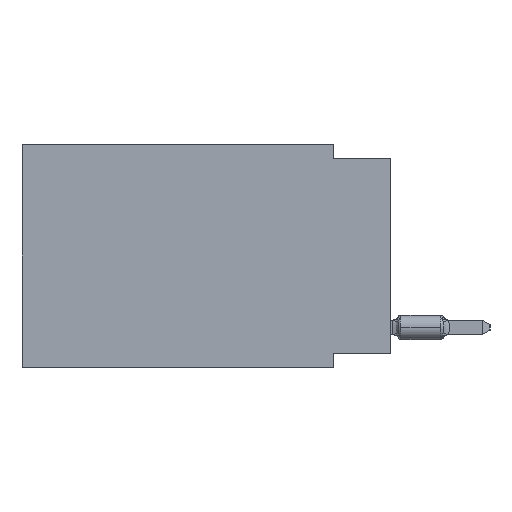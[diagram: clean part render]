
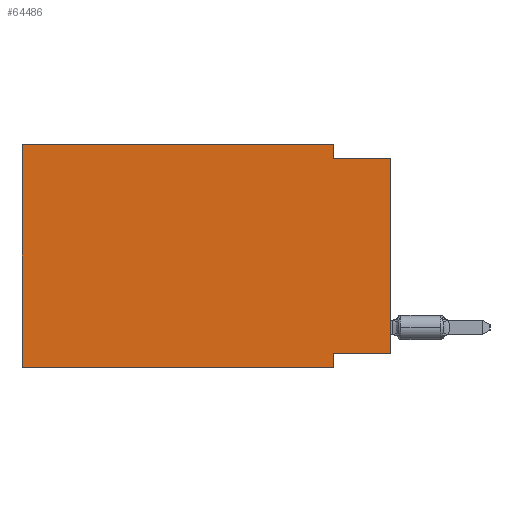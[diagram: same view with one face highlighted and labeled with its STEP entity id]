
A CAD part, left-side view. The second image highlights one B-rep face of the part: STEP entity #64486.
In plain terms, the highlighted planar face has unit normal (-1, 0, 0).
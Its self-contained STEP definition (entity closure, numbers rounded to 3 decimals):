
#163 = ORIENTED_EDGE ( 'NONE', *, *, #9097, .T. ) ;
#1084 = DIRECTION ( 'NONE',  ( 0., 0., -1. ) ) ;
#2475 = CARTESIAN_POINT ( 'NONE',  ( 0., 16.383, 0. ) ) ;
#3924 = ORIENTED_EDGE ( 'NONE', *, *, #72023, .T. ) ;
#7364 = FACE_OUTER_BOUND ( 'NONE', #16322, .T. ) ;
#7614 = VECTOR ( 'NONE', #77709, 1000. ) ;
#9097 = EDGE_CURVE ( 'NONE', #59812, #36264, #72421, .T. ) ;
#9628 = CARTESIAN_POINT ( 'NONE',  ( 0., 16.383, -9.906 ) ) ;
#10340 = LINE ( 'NONE', #39433, #47656 ) ;
#10862 = VERTEX_POINT ( 'NONE', #9628 ) ;
#11326 = VECTOR ( 'NONE', #39834, 1000. ) ;
#13310 = LINE ( 'NONE', #51734, #78958 ) ;
#13943 = DIRECTION ( 'NONE',  ( 0., -1., 0. ) ) ;
#14338 = CARTESIAN_POINT ( 'NONE',  ( 0., 0., 0. ) ) ;
#14536 = VERTEX_POINT ( 'NONE', #62178 ) ;
#16322 = EDGE_LOOP ( 'NONE', ( #163, #16633, #67341, #17047, #68066, #3924, #35411, #59381 ) ) ;
#16633 = ORIENTED_EDGE ( 'NONE', *, *, #61221, .F. ) ;
#17047 = ORIENTED_EDGE ( 'NONE', *, *, #76328, .F. ) ;
#17066 = CARTESIAN_POINT ( 'NONE',  ( 0., 16.383, 0. ) ) ;
#17553 = CARTESIAN_POINT ( 'NONE',  ( 0., 2.54, -0.635 ) ) ;
#19028 = AXIS2_PLACEMENT_3D ( 'NONE', #58326, #26972, #1084 ) ;
#21614 = VECTOR ( 'NONE', #68458, 1000. ) ;
#22104 = LINE ( 'NONE', #48428, #37806 ) ;
#25601 = LINE ( 'NONE', #38976, #79443 ) ;
#26600 = EDGE_CURVE ( 'NONE', #43666, #71563, #41132, .T. ) ;
#26709 = LINE ( 'NONE', #2475, #7614 ) ;
#26972 = DIRECTION ( 'NONE',  ( 1., 0., 0. ) ) ;
#31467 = CARTESIAN_POINT ( 'NONE',  ( 0., 2.54, 0. ) ) ;
#32695 = DIRECTION ( 'NONE',  ( 0., 0., -1. ) ) ;
#32841 = PLANE ( 'NONE',  #19028 ) ;
#35411 = ORIENTED_EDGE ( 'NONE', *, *, #35638, .F. ) ;
#35638 = EDGE_CURVE ( 'NONE', #73497, #14536, #25601, .T. ) ;
#36264 = VERTEX_POINT ( 'NONE', #61812 ) ;
#37806 = VECTOR ( 'NONE', #54695, 1000. ) ;
#38976 = CARTESIAN_POINT ( 'NONE',  ( 0., 2.54, -9.906 ) ) ;
#39433 = CARTESIAN_POINT ( 'NONE',  ( 0., 16.383, -9.906 ) ) ;
#39834 = DIRECTION ( 'NONE',  ( 0., 0., 1. ) ) ;
#41132 = LINE ( 'NONE', #66633, #49855 ) ;
#43666 = VERTEX_POINT ( 'NONE', #31467 ) ;
#45483 = EDGE_CURVE ( 'NONE', #59812, #73497, #22104, .T. ) ;
#47656 = VECTOR ( 'NONE', #13943, 1000. ) ;
#47749 = CARTESIAN_POINT ( 'NONE',  ( 0., 16.383, 0. ) ) ;
#48428 = CARTESIAN_POINT ( 'NONE',  ( 0., 0., -9.271 ) ) ;
#49855 = VECTOR ( 'NONE', #55741, 1000. ) ;
#51734 = CARTESIAN_POINT ( 'NONE',  ( 0., 0., -0.635 ) ) ;
#54695 = DIRECTION ( 'NONE',  ( 0., 1., 0. ) ) ;
#55138 = VERTEX_POINT ( 'NONE', #47749 ) ;
#55741 = DIRECTION ( 'NONE',  ( 0., 0., -1. ) ) ;
#57193 = EDGE_CURVE ( 'NONE', #10862, #55138, #81409, .T. ) ;
#58326 = CARTESIAN_POINT ( 'NONE',  ( 0., 16.383, 0. ) ) ;
#59381 = ORIENTED_EDGE ( 'NONE', *, *, #45483, .F. ) ;
#59812 = VERTEX_POINT ( 'NONE', #67249 ) ;
#61221 = EDGE_CURVE ( 'NONE', #71563, #36264, #13310, .T. ) ;
#61812 = CARTESIAN_POINT ( 'NONE',  ( 0., 0., -0.635 ) ) ;
#62178 = CARTESIAN_POINT ( 'NONE',  ( 0., 2.54, -9.906 ) ) ;
#64486 = ADVANCED_FACE ( 'NONE', ( #7364 ), #32841, .F. ) ;
#66633 = CARTESIAN_POINT ( 'NONE',  ( 0., 2.54, 0. ) ) ;
#67249 = CARTESIAN_POINT ( 'NONE',  ( 0., 0., -9.271 ) ) ;
#67341 = ORIENTED_EDGE ( 'NONE', *, *, #26600, .F. ) ;
#68066 = ORIENTED_EDGE ( 'NONE', *, *, #57193, .F. ) ;
#68458 = DIRECTION ( 'NONE',  ( 0., 0., 1. ) ) ;
#70565 = DIRECTION ( 'NONE',  ( 0., -1., 0. ) ) ;
#71108 = CARTESIAN_POINT ( 'NONE',  ( 0., 2.54, -9.271 ) ) ;
#71563 = VERTEX_POINT ( 'NONE', #17553 ) ;
#72023 = EDGE_CURVE ( 'NONE', #10862, #14536, #10340, .T. ) ;
#72421 = LINE ( 'NONE', #14338, #11326 ) ;
#73497 = VERTEX_POINT ( 'NONE', #71108 ) ;
#76328 = EDGE_CURVE ( 'NONE', #55138, #43666, #26709, .T. ) ;
#77709 = DIRECTION ( 'NONE',  ( 0., -1., 0. ) ) ;
#78958 = VECTOR ( 'NONE', #70565, 1000. ) ;
#79443 = VECTOR ( 'NONE', #32695, 1000. ) ;
#81409 = LINE ( 'NONE', #17066, #21614 ) ;
